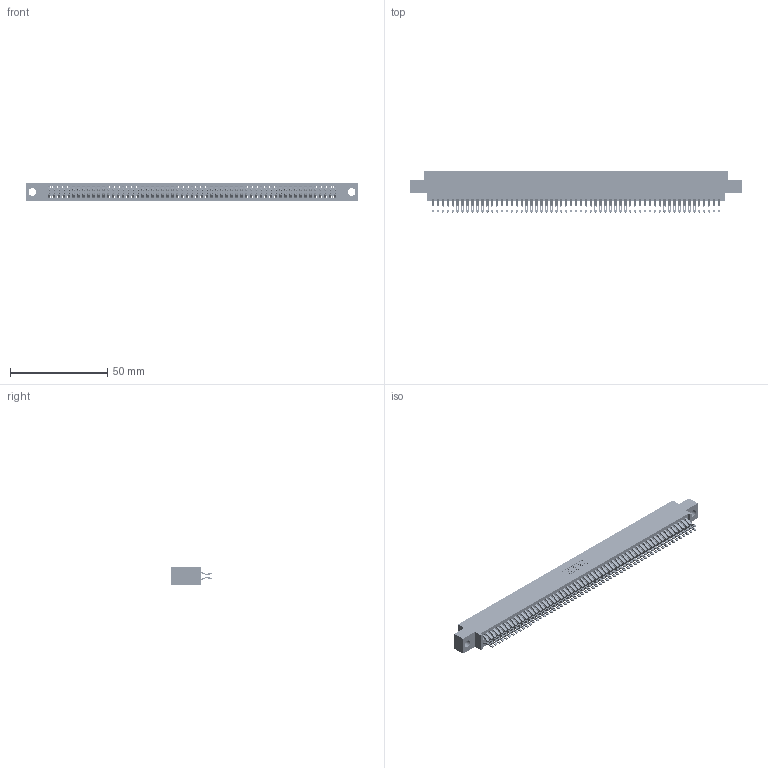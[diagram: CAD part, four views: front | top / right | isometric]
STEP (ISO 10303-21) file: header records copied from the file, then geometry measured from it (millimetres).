
FILE_DESCRIPTION (( 'STEP AP203' ), '1' );
FILE_NAME ('345-118-555-804.STEP', '2021-05-25T16:28:00', ( '' ), ( '' ), 'SwSTEP 2.0', 'SolidWorks 2020', '' );
FILE_SCHEMA (( 'CONFIG_CONTROL_DESIGN' ));
Length unit declared in the file: inch
Products named in the file (3): 345-292-001_555 Tail; 345 Part_0.170 Offset - 0.156 Dia-TI; 345-118-555-804
Assembly tree (119 placements, depth 2):
  345-118-555-804
    345 Part_0.170 Offset - 0.156 Dia-TI
    345-292-001_555 Tail  x118
Bounding box: 171.07 x 21.13 x 9.4 mm (x, y, z)
Volume: 16898.5 mm3; surface area: 26493.6 mm2
Topology: 119 solids, 119 shells, 6752 faces, 21275 edges, 14182 vertices
Faces by surface type: plane 3756, cylinder 2996
Entity records: 44881 total; most frequent: CARTESIAN_POINT 7548, ORIENTED_EDGE 7450, DIRECTION 6601, EDGE_CURVE 3725, VECTOR 3337, LINE 3337, VERTEX_POINT 2482, AXIS2_PLACEMENT_3D 1632
